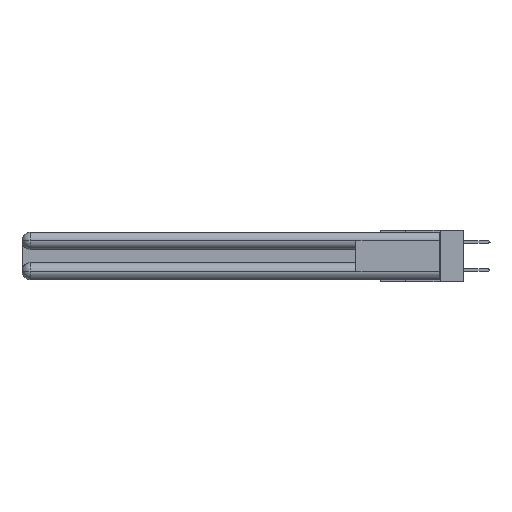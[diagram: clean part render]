
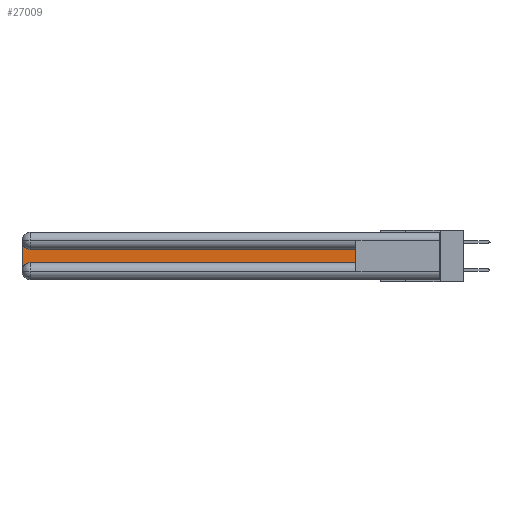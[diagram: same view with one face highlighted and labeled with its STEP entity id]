
A CAD part, left-side view. The second image highlights one B-rep face of the part: STEP entity #27009.
In plain terms, the highlighted planar face has unit normal (-1, 0, 0).
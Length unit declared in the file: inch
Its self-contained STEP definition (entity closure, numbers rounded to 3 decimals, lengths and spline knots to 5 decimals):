
#555 = CARTESIAN_POINT ( 'NONE',  ( 0.075, 0.6, -0.2175 ) ) ;
#603 = DIRECTION ( 'NONE',  ( 0., 0., -1. ) ) ;
#898 = EDGE_CURVE ( 'NONE', #26355, #4219, #14598, .T. ) ;
#2201 = DIRECTION ( 'NONE',  ( 0., 0., 1. ) ) ;
#2289 = ORIENTED_EDGE ( 'NONE', *, *, #7562, .T. ) ;
#2306 = EDGE_CURVE ( 'NONE', #6531, #9451, #24591, .T. ) ;
#2381 = CARTESIAN_POINT ( 'NONE',  ( 0.075, 0.6, -0.2175 ) ) ;
#2578 = VERTEX_POINT ( 'NONE', #11442 ) ;
#2863 = DIRECTION ( 'NONE',  ( 0., 0., -1. ) ) ;
#3676 = AXIS2_PLACEMENT_3D ( 'NONE', #21638, #13291, #603 ) ;
#4167 = CARTESIAN_POINT ( 'NONE',  ( 0.075, 0.6, -0.1225 ) ) ;
#4219 = VERTEX_POINT ( 'NONE', #5373 ) ;
#4289 = ORIENTED_EDGE ( 'NONE', *, *, #8271, .T. ) ;
#5373 = CARTESIAN_POINT ( 'NONE',  ( 0.075, 3., -0.0625 ) ) ;
#6531 = VERTEX_POINT ( 'NONE', #24157 ) ;
#7555 = CARTESIAN_POINT ( 'NONE',  ( 0.075, 0.6, -0.1225 ) ) ;
#7562 = EDGE_CURVE ( 'NONE', #2578, #6531, #16061, .T. ) ;
#7990 = DIRECTION ( 'NONE',  ( 0., 0., -1. ) ) ;
#8271 = EDGE_CURVE ( 'NONE', #8704, #26355, #8328, .T. ) ;
#8328 = LINE ( 'NONE', #7555, #19434 ) ;
#8422 = ORIENTED_EDGE ( 'NONE', *, *, #898, .T. ) ;
#8704 = VERTEX_POINT ( 'NONE', #4167 ) ;
#8896 = DIRECTION ( 'NONE',  ( 0., -1., 0. ) ) ;
#9451 = VERTEX_POINT ( 'NONE', #16978 ) ;
#10748 = CARTESIAN_POINT ( 'NONE',  ( 0.075, 2.94, -0.0625 ) ) ;
#11114 = PLANE ( 'NONE',  #3676 ) ;
#11156 = VECTOR ( 'NONE', #8896, 39.37008 ) ;
#11442 = CARTESIAN_POINT ( 'NONE',  ( 0.075, 3., -0.2775 ) ) ;
#12105 = ORIENTED_EDGE ( 'NONE', *, *, #22204, .T. ) ;
#12180 = AXIS2_PLACEMENT_3D ( 'NONE', #10748, #12730, #19327 ) ;
#12730 = DIRECTION ( 'NONE',  ( 1., 0., 0. ) ) ;
#13216 = DIRECTION ( 'NONE',  ( 1., 0., 0. ) ) ;
#13291 = DIRECTION ( 'NONE',  ( 1., 0., 0. ) ) ;
#13298 = ORIENTED_EDGE ( 'NONE', *, *, #18106, .T. ) ;
#14210 = CARTESIAN_POINT ( 'NONE',  ( 0.075, 3., -0.2175 ) ) ;
#14598 = CIRCLE ( 'NONE', #12180, 0.06 ) ;
#15648 = CARTESIAN_POINT ( 'NONE',  ( 0.075, 2.94, -0.2775 ) ) ;
#15752 = CARTESIAN_POINT ( 'NONE',  ( 0.075, 2.94, -0.1225 ) ) ;
#16061 = CIRCLE ( 'NONE', #24869, 0.06 ) ;
#16186 = DIRECTION ( 'NONE',  ( 0., 1., 0. ) ) ;
#16978 = CARTESIAN_POINT ( 'NONE',  ( 0.075, 0.6, -0.2175 ) ) ;
#17131 = ORIENTED_EDGE ( 'NONE', *, *, #2306, .T. ) ;
#18106 = EDGE_CURVE ( 'NONE', #9451, #8704, #22063, .T. ) ;
#19327 = DIRECTION ( 'NONE',  ( 0., 0., -1. ) ) ;
#19434 = VECTOR ( 'NONE', #16186, 39.37008 ) ;
#21638 = CARTESIAN_POINT ( 'NONE',  ( 0.075, 3., -0.1225 ) ) ;
#22063 = LINE ( 'NONE', #2381, #23066 ) ;
#22204 = EDGE_CURVE ( 'NONE', #4219, #2578, #26076, .T. ) ;
#23042 = VECTOR ( 'NONE', #7990, 39.37008 ) ;
#23066 = VECTOR ( 'NONE', #2201, 39.37008 ) ;
#23865 = EDGE_LOOP ( 'NONE', ( #4289, #8422, #12105, #2289, #17131, #13298 ) ) ;
#24157 = CARTESIAN_POINT ( 'NONE',  ( 0.075, 2.94, -0.2175 ) ) ;
#24591 = LINE ( 'NONE', #555, #11156 ) ;
#24869 = AXIS2_PLACEMENT_3D ( 'NONE', #15648, #13216, #2863 ) ;
#25526 = FACE_OUTER_BOUND ( 'NONE', #23865, .T. ) ;
#26076 = LINE ( 'NONE', #14210, #23042 ) ;
#26355 = VERTEX_POINT ( 'NONE', #15752 ) ;
#27009 = ADVANCED_FACE ( 'NONE', ( #25526 ), #11114, .F. ) ;
